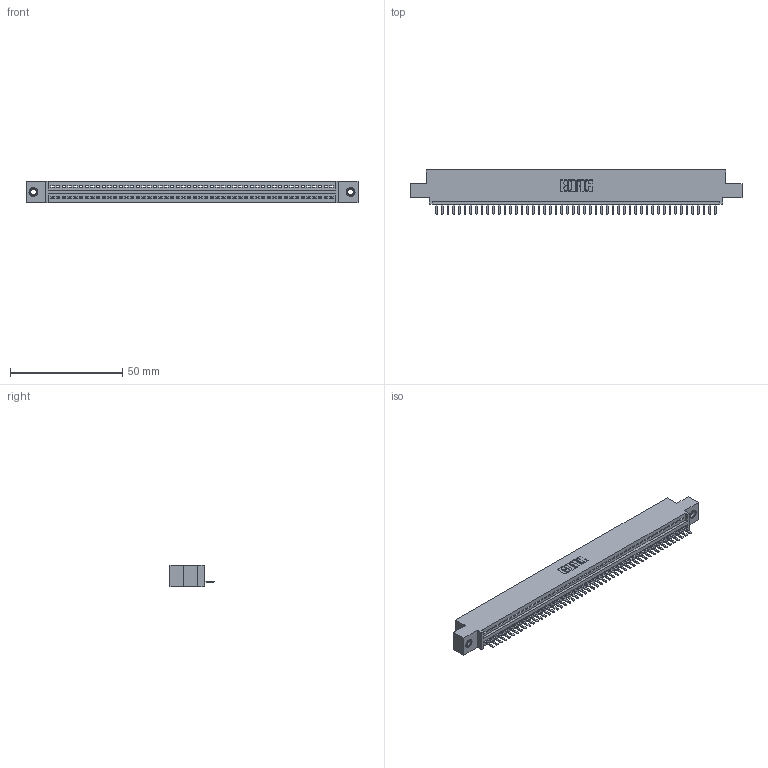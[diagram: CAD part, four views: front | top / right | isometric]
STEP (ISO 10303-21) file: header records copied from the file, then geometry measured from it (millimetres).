
FILE_DESCRIPTION (( 'STEP AP203' ), '1' );
FILE_NAME ('345-050-520-407.STEP', '2019-10-09T10:41:51', ( '' ), ( '' ), 'SwSTEP 2.0', 'SolidWorks 2016', '' );
FILE_SCHEMA (( 'CONFIG_CONTROL_DESIGN' ));
Length unit declared in the file: inch
Products named in the file (4): 345 Part_0.110 Offset - 0.156 Dia-TI; 345-050-520-407; 345-292-001_345-293-120; 345-250-001_345-250-005-103
Assembly tree (53 placements, depth 2):
  345-050-520-407
    345 Part_0.110 Offset - 0.156 Dia-TI
    345-292-001_345-293-120  x50
    345-250-001_345-250-005-103  x2
Bounding box: 148.21 x 19.68 x 9.4 mm (x, y, z)
Volume: 13911.9 mm3; surface area: 18240.3 mm2
Topology: 53 solids, 53 shells, 3290 faces, 9689 edges, 6318 vertices
Faces by surface type: plane 2216, cylinder 1058, cone 12, torus 4
Entity records: 37986 total; most frequent: CARTESIAN_POINT 6573, ORIENTED_EDGE 6538, DIRECTION 5743, EDGE_CURVE 3269, VECTOR 2913, LINE 2913, VERTEX_POINT 2172, AXIS2_PLACEMENT_3D 1415
